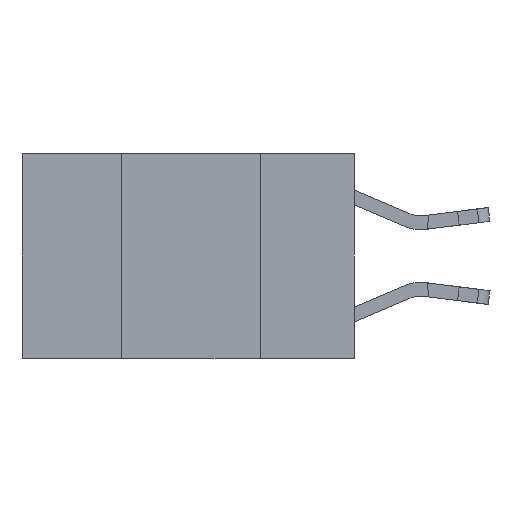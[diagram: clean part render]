
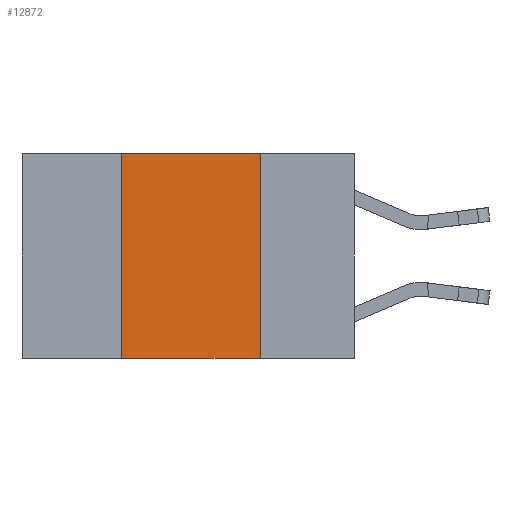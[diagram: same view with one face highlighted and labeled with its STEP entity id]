
A CAD part, left-side view. The second image highlights one B-rep face of the part: STEP entity #12872.
In plain terms, the highlighted planar face has unit normal (-1, 0, 0).
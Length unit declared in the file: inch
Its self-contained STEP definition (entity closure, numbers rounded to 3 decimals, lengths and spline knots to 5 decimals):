
#33 = ORIENTED_EDGE ( 'NONE', *, *, #13065, .T. ) ;
#194 = ORIENTED_EDGE ( 'NONE', *, *, #8137, .F. ) ;
#398 = EDGE_LOOP ( 'NONE', ( #2730, #194, #1220, #33 ) ) ;
#736 = DIRECTION ( 'NONE',  ( 0., 0., -1. ) ) ;
#1220 = ORIENTED_EDGE ( 'NONE', *, *, #10364, .F. ) ;
#1226 = VECTOR ( 'NONE', #9740, 39.37008 ) ;
#1384 = VERTEX_POINT ( 'NONE', #6697 ) ;
#1560 = LINE ( 'NONE', #8632, #1226 ) ;
#2489 = LINE ( 'NONE', #8116, #13326 ) ;
#2730 = ORIENTED_EDGE ( 'NONE', *, *, #8244, .F. ) ;
#3666 = VECTOR ( 'NONE', #6084, 39.37008 ) ;
#4915 = DIRECTION ( 'NONE',  ( 0., -1., 0. ) ) ;
#6084 = DIRECTION ( 'NONE',  ( 0., 0., -1. ) ) ;
#6112 = PLANE ( 'NONE',  #8611 ) ;
#6697 = CARTESIAN_POINT ( 'NONE',  ( 0., 0.42, 0. ) ) ;
#7202 = DIRECTION ( 'NONE',  ( 1., 0., 0. ) ) ;
#8116 = CARTESIAN_POINT ( 'NONE',  ( 0., 0.6, 0. ) ) ;
#8137 = EDGE_CURVE ( 'NONE', #1384, #12455, #2489, .T. ) ;
#8244 = EDGE_CURVE ( 'NONE', #12455, #10329, #12296, .T. ) ;
#8611 = AXIS2_PLACEMENT_3D ( 'NONE', #13721, #7202, #736 ) ;
#8632 = CARTESIAN_POINT ( 'NONE',  ( 0., 0.6, -0.37 ) ) ;
#8696 = CARTESIAN_POINT ( 'NONE',  ( 0., 0.17, 0. ) ) ;
#8850 = LINE ( 'NONE', #10176, #9208 ) ;
#9208 = VECTOR ( 'NONE', #11255, 39.37008 ) ;
#9656 = VERTEX_POINT ( 'NONE', #12261 ) ;
#9699 = FACE_OUTER_BOUND ( 'NONE', #398, .T. ) ;
#9740 = DIRECTION ( 'NONE',  ( 0., -1., 0. ) ) ;
#10129 = CARTESIAN_POINT ( 'NONE',  ( 0., 0.17, -0.37 ) ) ;
#10176 = CARTESIAN_POINT ( 'NONE',  ( 0., 0.42, 0. ) ) ;
#10329 = VERTEX_POINT ( 'NONE', #10129 ) ;
#10364 = EDGE_CURVE ( 'NONE', #9656, #1384, #8850, .T. ) ;
#10462 = CARTESIAN_POINT ( 'NONE',  ( 0., 0.17, 0. ) ) ;
#11255 = DIRECTION ( 'NONE',  ( 0., 0., 1. ) ) ;
#12261 = CARTESIAN_POINT ( 'NONE',  ( 0., 0.42, -0.37 ) ) ;
#12296 = LINE ( 'NONE', #10462, #3666 ) ;
#12455 = VERTEX_POINT ( 'NONE', #8696 ) ;
#12872 = ADVANCED_FACE ( 'NONE', ( #9699 ), #6112, .F. ) ;
#13065 = EDGE_CURVE ( 'NONE', #9656, #10329, #1560, .T. ) ;
#13326 = VECTOR ( 'NONE', #4915, 39.37008 ) ;
#13721 = CARTESIAN_POINT ( 'NONE',  ( 0., 0.6, 0. ) ) ;
